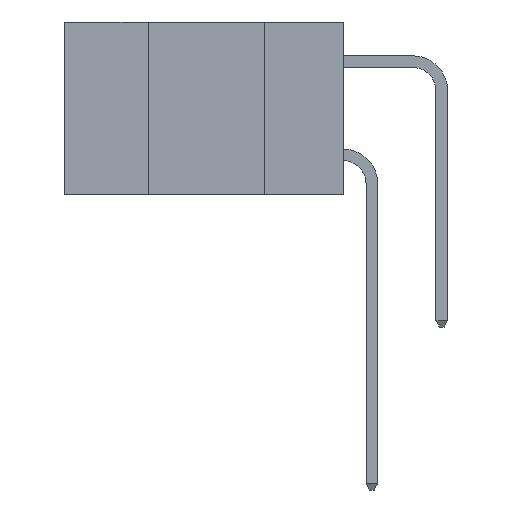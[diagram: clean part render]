
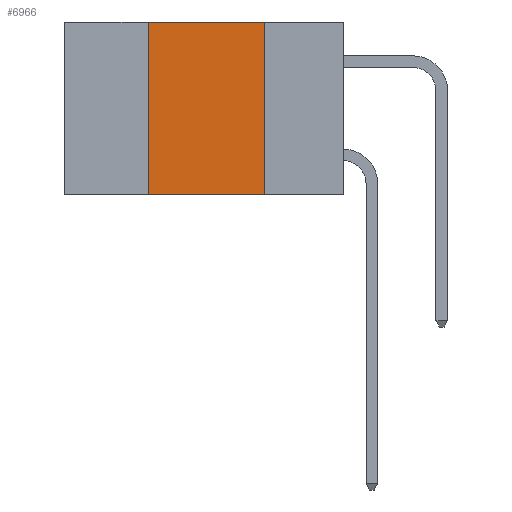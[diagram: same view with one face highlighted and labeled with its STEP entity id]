
A CAD part, left-side view. The second image highlights one B-rep face of the part: STEP entity #6966.
In plain terms, the highlighted planar face has unit normal (-1, 0, 0).
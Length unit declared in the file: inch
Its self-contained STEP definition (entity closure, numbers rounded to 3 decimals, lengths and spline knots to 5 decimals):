
#276 = LINE ( 'NONE', #7673, #14158 ) ;
#394 = ORIENTED_EDGE ( 'NONE', *, *, #4042, .F. ) ;
#1049 = DIRECTION ( 'NONE',  ( 0., 0., 1. ) ) ;
#1193 = AXIS2_PLACEMENT_3D ( 'NONE', #1672, #10555, #3994 ) ;
#1244 = ORIENTED_EDGE ( 'NONE', *, *, #4508, .T. ) ;
#1539 = CARTESIAN_POINT ( 'NONE',  ( 0., 0.17, -0.37 ) ) ;
#1627 = VERTEX_POINT ( 'NONE', #8843 ) ;
#1672 = CARTESIAN_POINT ( 'NONE',  ( 0., 0.6, 0. ) ) ;
#1684 = EDGE_LOOP ( 'NONE', ( #394, #10302, #2877, #1244 ) ) ;
#1747 = CARTESIAN_POINT ( 'NONE',  ( 0., 0.6, -0.37 ) ) ;
#2107 = VECTOR ( 'NONE', #12007, 39.37008 ) ;
#2849 = PLANE ( 'NONE',  #1193 ) ;
#2877 = ORIENTED_EDGE ( 'NONE', *, *, #5961, .F. ) ;
#3120 = VERTEX_POINT ( 'NONE', #1539 ) ;
#3994 = DIRECTION ( 'NONE',  ( 0., 0., -1. ) ) ;
#4042 = EDGE_CURVE ( 'NONE', #8841, #3120, #7612, .T. ) ;
#4375 = CARTESIAN_POINT ( 'NONE',  ( 0., 0.17, -0.37 ) ) ;
#4487 = DIRECTION ( 'NONE',  ( 0., -1., 0. ) ) ;
#4508 = EDGE_CURVE ( 'NONE', #12816, #3120, #4716, .T. ) ;
#4716 = LINE ( 'NONE', #1747, #7958 ) ;
#4860 = CARTESIAN_POINT ( 'NONE',  ( 0., 0.17, 0. ) ) ;
#5961 = EDGE_CURVE ( 'NONE', #12816, #1627, #276, .T. ) ;
#6000 = FACE_OUTER_BOUND ( 'NONE', #1684, .T. ) ;
#6693 = EDGE_CURVE ( 'NONE', #1627, #8841, #12337, .T. ) ;
#6966 = ADVANCED_FACE ( 'NONE', ( #6000 ), #2849, .F. ) ;
#7612 = LINE ( 'NONE', #4375, #2107 ) ;
#7673 = CARTESIAN_POINT ( 'NONE',  ( 0., 0.42, -0.37 ) ) ;
#7958 = VECTOR ( 'NONE', #8355, 39.37008 ) ;
#8355 = DIRECTION ( 'NONE',  ( 0., -1., 0. ) ) ;
#8841 = VERTEX_POINT ( 'NONE', #4860 ) ;
#8843 = CARTESIAN_POINT ( 'NONE',  ( 0., 0.42, 0. ) ) ;
#9412 = VECTOR ( 'NONE', #4487, 39.37008 ) ;
#9914 = CARTESIAN_POINT ( 'NONE',  ( 0., 0.6, 0. ) ) ;
#10302 = ORIENTED_EDGE ( 'NONE', *, *, #6693, .F. ) ;
#10555 = DIRECTION ( 'NONE',  ( 1., 0., 0. ) ) ;
#12007 = DIRECTION ( 'NONE',  ( 0., 0., -1. ) ) ;
#12158 = CARTESIAN_POINT ( 'NONE',  ( 0., 0.42, -0.37 ) ) ;
#12337 = LINE ( 'NONE', #9914, #9412 ) ;
#12816 = VERTEX_POINT ( 'NONE', #12158 ) ;
#14158 = VECTOR ( 'NONE', #1049, 39.37008 ) ;
